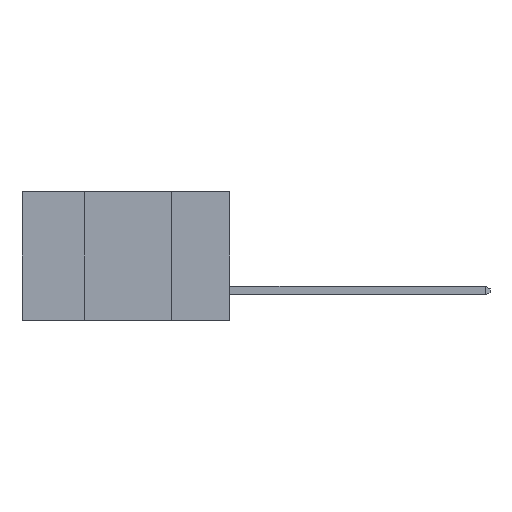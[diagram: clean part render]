
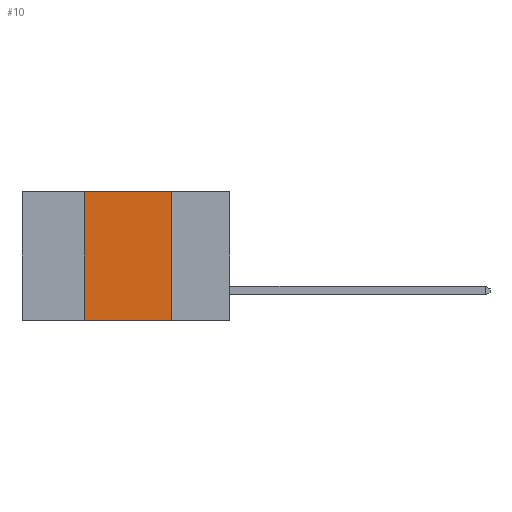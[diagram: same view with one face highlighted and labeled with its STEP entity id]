
A CAD part, left-side view. The second image highlights one B-rep face of the part: STEP entity #10.
In plain terms, the highlighted planar face has unit normal (-1, 0, 0).
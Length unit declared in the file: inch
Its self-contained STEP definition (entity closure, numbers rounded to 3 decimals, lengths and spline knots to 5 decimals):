
#10 = ADVANCED_FACE ( 'NONE', ( #9458 ), #11693, .F. ) ;
#1704 = EDGE_LOOP ( 'NONE', ( #6258, #2716, #11471, #2217 ) ) ;
#1830 = LINE ( 'NONE', #12038, #2205 ) ;
#1993 = DIRECTION ( 'NONE',  ( 1., 0., 0. ) ) ;
#2205 = VECTOR ( 'NONE', #5578, 39.37008 ) ;
#2217 = ORIENTED_EDGE ( 'NONE', *, *, #12222, .T. ) ;
#2487 = EDGE_CURVE ( 'NONE', #3417, #10966, #1830, .T. ) ;
#2716 = ORIENTED_EDGE ( 'NONE', *, *, #11038, .F. ) ;
#2966 = LINE ( 'NONE', #11185, #6044 ) ;
#3143 = DIRECTION ( 'NONE',  ( 0., 0., -1. ) ) ;
#3249 = CARTESIAN_POINT ( 'NONE',  ( 0., 0.6, 0. ) ) ;
#3417 = VERTEX_POINT ( 'NONE', #12938 ) ;
#3529 = DIRECTION ( 'NONE',  ( 0., -1., 0. ) ) ;
#5031 = VERTEX_POINT ( 'NONE', #11828 ) ;
#5429 = VERTEX_POINT ( 'NONE', #12092 ) ;
#5578 = DIRECTION ( 'NONE',  ( 0., 0., -1. ) ) ;
#6044 = VECTOR ( 'NONE', #12292, 39.37008 ) ;
#6258 = ORIENTED_EDGE ( 'NONE', *, *, #2487, .F. ) ;
#6706 = CARTESIAN_POINT ( 'NONE',  ( 0., 0.42, -0.37 ) ) ;
#6949 = LINE ( 'NONE', #3249, #12015 ) ;
#7350 = EDGE_CURVE ( 'NONE', #5031, #5429, #8566, .T. ) ;
#8082 = AXIS2_PLACEMENT_3D ( 'NONE', #8579, #1993, #3143 ) ;
#8566 = LINE ( 'NONE', #6706, #12458 ) ;
#8579 = CARTESIAN_POINT ( 'NONE',  ( 0., 0.6, 0. ) ) ;
#9458 = FACE_OUTER_BOUND ( 'NONE', #1704, .T. ) ;
#10966 = VERTEX_POINT ( 'NONE', #11525 ) ;
#11038 = EDGE_CURVE ( 'NONE', #5429, #3417, #6949, .T. ) ;
#11185 = CARTESIAN_POINT ( 'NONE',  ( 0., 0.6, -0.37 ) ) ;
#11471 = ORIENTED_EDGE ( 'NONE', *, *, #7350, .F. ) ;
#11525 = CARTESIAN_POINT ( 'NONE',  ( 0., 0.17, -0.37 ) ) ;
#11693 = PLANE ( 'NONE',  #8082 ) ;
#11828 = CARTESIAN_POINT ( 'NONE',  ( 0., 0.42, -0.37 ) ) ;
#12015 = VECTOR ( 'NONE', #3529, 39.37008 ) ;
#12038 = CARTESIAN_POINT ( 'NONE',  ( 0., 0.17, -0.37 ) ) ;
#12092 = CARTESIAN_POINT ( 'NONE',  ( 0., 0.42, 0. ) ) ;
#12222 = EDGE_CURVE ( 'NONE', #5031, #10966, #2966, .T. ) ;
#12292 = DIRECTION ( 'NONE',  ( 0., -1., 0. ) ) ;
#12458 = VECTOR ( 'NONE', #13026, 39.37008 ) ;
#12938 = CARTESIAN_POINT ( 'NONE',  ( 0., 0.17, 0. ) ) ;
#13026 = DIRECTION ( 'NONE',  ( 0., 0., 1. ) ) ;
